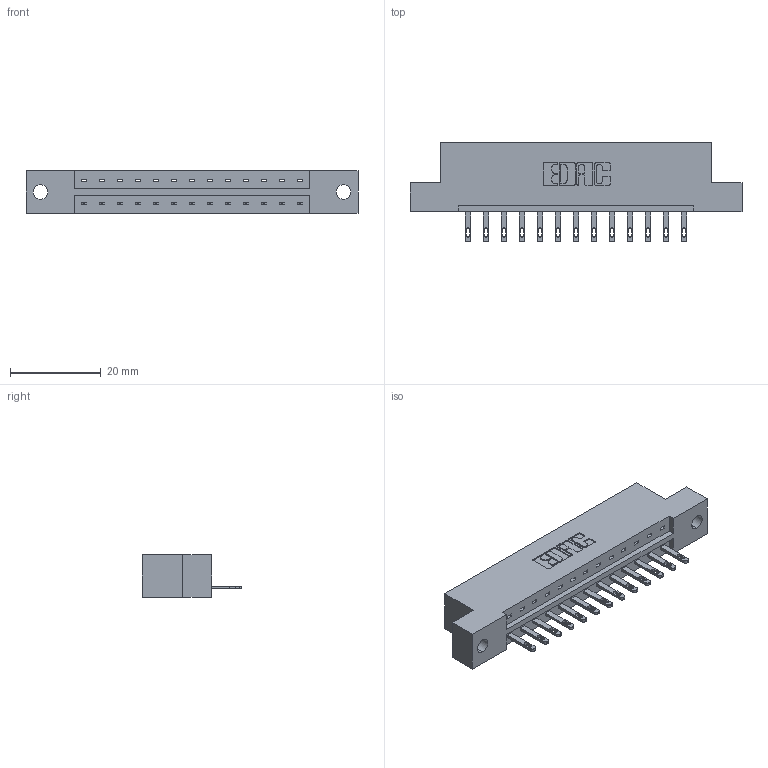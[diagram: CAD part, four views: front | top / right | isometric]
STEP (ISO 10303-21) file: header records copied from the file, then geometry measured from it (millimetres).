
FILE_DESCRIPTION (( 'STEP AP203' ), '1' );
FILE_NAME ('833-013-500-102.STEP', '2020-05-30T23:22:31', ( '' ), ( '' ), 'SwSTEP 2.0', 'SolidWorks 2020', '' );
FILE_SCHEMA (( 'CONFIG_CONTROL_DESIGN' ));
Length unit declared in the file: inch
Products named in the file (3): 345-292-001_345-293-100; 833 Part_Flush - .128 Dia; 833-013-500-102
Assembly tree (14 placements, depth 2):
  833-013-500-102
    833 Part_Flush - .128 Dia
    345-292-001_345-293-100  x13
Bounding box: 73.05 x 21.85 x 9.4 mm (x, y, z)
Volume: 7072.9 mm3; surface area: 7222.2 mm2
Topology: 14 solids, 14 shells, 816 faces, 2495 edges, 1662 vertices
Faces by surface type: plane 538, cylinder 278
Entity records: 11631 total; most frequent: CARTESIAN_POINT 2017, ORIENTED_EDGE 1966, DIRECTION 1761, EDGE_CURVE 983, LINE 851, VECTOR 851, VERTEX_POINT 654, AXIS2_PLACEMENT_3D 455
